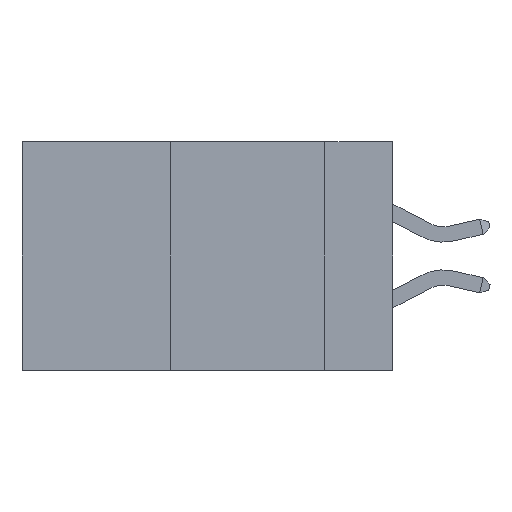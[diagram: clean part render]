
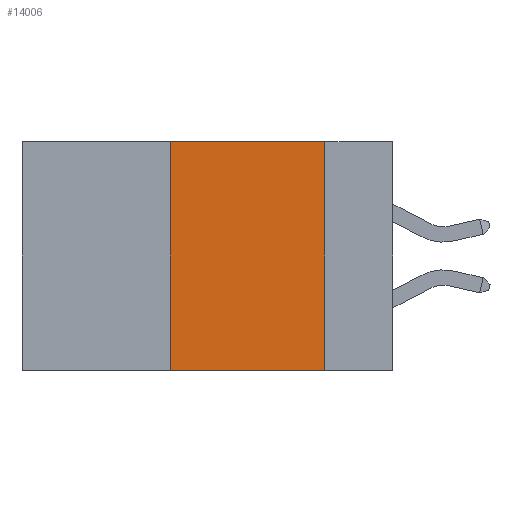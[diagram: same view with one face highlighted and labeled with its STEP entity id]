
A CAD part, left-side view. The second image highlights one B-rep face of the part: STEP entity #14006.
In plain terms, the highlighted planar face has unit normal (-1, 0, 0).
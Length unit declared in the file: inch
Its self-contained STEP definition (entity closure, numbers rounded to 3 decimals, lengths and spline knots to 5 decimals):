
#154 = EDGE_CURVE ( 'NONE', #1563, #28937, #8218, .T. ) ;
#754 = CARTESIAN_POINT ( 'NONE',  ( 0., 0.36, -0.37 ) ) ;
#1563 = VERTEX_POINT ( 'NONE', #19131 ) ;
#2964 = CARTESIAN_POINT ( 'NONE',  ( 0., 0.11, 0. ) ) ;
#7636 = DIRECTION ( 'NONE',  ( 0., 0., 1. ) ) ;
#7861 = DIRECTION ( 'NONE',  ( 0., 0., -1. ) ) ;
#8218 = LINE ( 'NONE', #2964, #32573 ) ;
#8966 = LINE ( 'NONE', #13544, #11466 ) ;
#10640 = CARTESIAN_POINT ( 'NONE',  ( 0., 0.11, -0.37 ) ) ;
#10966 = CARTESIAN_POINT ( 'NONE',  ( 0., 0.36, 0. ) ) ;
#11466 = VECTOR ( 'NONE', #16589, 39.37008 ) ;
#11636 = EDGE_LOOP ( 'NONE', ( #27240, #34389, #31708, #14180 ) ) ;
#12067 = PLANE ( 'NONE',  #18933 ) ;
#12411 = DIRECTION ( 'NONE',  ( 0., 0., -1. ) ) ;
#13544 = CARTESIAN_POINT ( 'NONE',  ( 0., 0.6, -0.37 ) ) ;
#13554 = LINE ( 'NONE', #34866, #19488 ) ;
#14006 = ADVANCED_FACE ( 'NONE', ( #30717 ), #12067, .F. ) ;
#14180 = ORIENTED_EDGE ( 'NONE', *, *, #29628, .T. ) ;
#14905 = VERTEX_POINT ( 'NONE', #754 ) ;
#16056 = LINE ( 'NONE', #10966, #22022 ) ;
#16589 = DIRECTION ( 'NONE',  ( 0., -1., 0. ) ) ;
#18876 = CARTESIAN_POINT ( 'NONE',  ( 0., 0.6, 0. ) ) ;
#18933 = AXIS2_PLACEMENT_3D ( 'NONE', #18876, #21779, #7861 ) ;
#19131 = CARTESIAN_POINT ( 'NONE',  ( 0., 0.11, 0. ) ) ;
#19488 = VECTOR ( 'NONE', #37737, 39.37008 ) ;
#21421 = VERTEX_POINT ( 'NONE', #25933 ) ;
#21779 = DIRECTION ( 'NONE',  ( 1., 0., 0. ) ) ;
#22022 = VECTOR ( 'NONE', #7636, 39.37008 ) ;
#25933 = CARTESIAN_POINT ( 'NONE',  ( 0., 0.36, 0. ) ) ;
#26167 = EDGE_CURVE ( 'NONE', #21421, #1563, #13554, .T. ) ;
#27240 = ORIENTED_EDGE ( 'NONE', *, *, #154, .F. ) ;
#28937 = VERTEX_POINT ( 'NONE', #10640 ) ;
#29628 = EDGE_CURVE ( 'NONE', #14905, #28937, #8966, .T. ) ;
#30717 = FACE_OUTER_BOUND ( 'NONE', #11636, .T. ) ;
#31708 = ORIENTED_EDGE ( 'NONE', *, *, #39782, .F. ) ;
#32573 = VECTOR ( 'NONE', #12411, 39.37008 ) ;
#34389 = ORIENTED_EDGE ( 'NONE', *, *, #26167, .F. ) ;
#34866 = CARTESIAN_POINT ( 'NONE',  ( 0., 0.6, 0. ) ) ;
#37737 = DIRECTION ( 'NONE',  ( 0., -1., 0. ) ) ;
#39782 = EDGE_CURVE ( 'NONE', #14905, #21421, #16056, .T. ) ;
